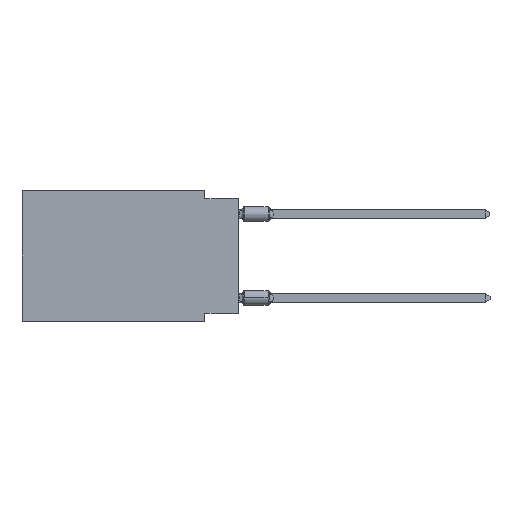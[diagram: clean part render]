
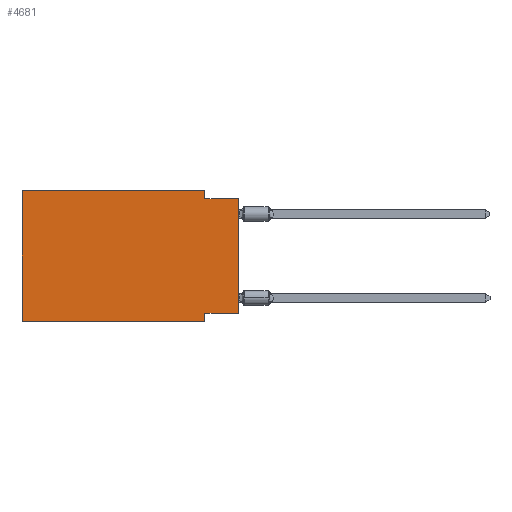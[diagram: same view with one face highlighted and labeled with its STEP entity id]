
A CAD part, left-side view. The second image highlights one B-rep face of the part: STEP entity #4681.
In plain terms, the highlighted planar face has unit normal (-1, 0, 0).
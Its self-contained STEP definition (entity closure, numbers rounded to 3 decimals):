
#393 = VECTOR ( 'NONE', #967, 1000. ) ;
#500 = DIRECTION ( 'NONE',  ( 0., 1., 0. ) ) ;
#753 = CARTESIAN_POINT ( 'NONE',  ( 0., 2.54, 0. ) ) ;
#770 = VECTOR ( 'NONE', #23218, 1000. ) ;
#847 = LINE ( 'NONE', #4519, #770 ) ;
#901 = CARTESIAN_POINT ( 'NONE',  ( 0., 0., -0.635 ) ) ;
#967 = DIRECTION ( 'NONE',  ( 0., -1., 0. ) ) ;
#1133 = VECTOR ( 'NONE', #22159, 1000. ) ;
#1694 = AXIS2_PLACEMENT_3D ( 'NONE', #12767, #22157, #8851 ) ;
#1802 = ORIENTED_EDGE ( 'NONE', *, *, #13417, .T. ) ;
#1824 = VECTOR ( 'NONE', #11027, 1000. ) ;
#2027 = ORIENTED_EDGE ( 'NONE', *, *, #6627, .F. ) ;
#2348 = LINE ( 'NONE', #753, #22731 ) ;
#2801 = LINE ( 'NONE', #17723, #393 ) ;
#3312 = CARTESIAN_POINT ( 'NONE',  ( 0., 16.383, -9.906 ) ) ;
#3412 = CARTESIAN_POINT ( 'NONE',  ( 0., 2.54, -9.906 ) ) ;
#3560 = CARTESIAN_POINT ( 'NONE',  ( 0., 2.54, 0. ) ) ;
#3595 = ORIENTED_EDGE ( 'NONE', *, *, #3862, .F. ) ;
#3862 = EDGE_CURVE ( 'NONE', #17677, #14740, #12739, .T. ) ;
#4302 = EDGE_CURVE ( 'NONE', #20389, #4439, #18160, .T. ) ;
#4439 = VERTEX_POINT ( 'NONE', #901 ) ;
#4519 = CARTESIAN_POINT ( 'NONE',  ( 0., 0., 0. ) ) ;
#4681 = ADVANCED_FACE ( 'NONE', ( #8731 ), #5280, .F. ) ;
#4986 = VERTEX_POINT ( 'NONE', #3312 ) ;
#5280 = PLANE ( 'NONE',  #1694 ) ;
#5672 = CARTESIAN_POINT ( 'NONE',  ( 0., 0., -0.635 ) ) ;
#6627 = EDGE_CURVE ( 'NONE', #17082, #17677, #20934, .T. ) ;
#7326 = CARTESIAN_POINT ( 'NONE',  ( 0., 2.54, -9.906 ) ) ;
#8063 = ORIENTED_EDGE ( 'NONE', *, *, #4302, .F. ) ;
#8145 = ORIENTED_EDGE ( 'NONE', *, *, #13452, .T. ) ;
#8538 = EDGE_LOOP ( 'NONE', ( #1802, #8063, #15615, #14293, #20192, #8145, #3595, #2027 ) ) ;
#8731 = FACE_OUTER_BOUND ( 'NONE', #8538, .T. ) ;
#8851 = DIRECTION ( 'NONE',  ( 0., 0., -1. ) ) ;
#9338 = CARTESIAN_POINT ( 'NONE',  ( 0., 16.383, 0. ) ) ;
#11027 = DIRECTION ( 'NONE',  ( 0., 0., -1. ) ) ;
#11295 = CARTESIAN_POINT ( 'NONE',  ( 0., 16.383, 0. ) ) ;
#11625 = VECTOR ( 'NONE', #500, 1000. ) ;
#11917 = EDGE_CURVE ( 'NONE', #14291, #20389, #2348, .T. ) ;
#12386 = CARTESIAN_POINT ( 'NONE',  ( 0., 16.383, 0. ) ) ;
#12739 = LINE ( 'NONE', #7326, #1824 ) ;
#12767 = CARTESIAN_POINT ( 'NONE',  ( 0., 16.383, 0. ) ) ;
#13256 = LINE ( 'NONE', #9338, #14439 ) ;
#13417 = EDGE_CURVE ( 'NONE', #17082, #4439, #847, .T. ) ;
#13452 = EDGE_CURVE ( 'NONE', #4986, #14740, #2801, .T. ) ;
#13636 = CARTESIAN_POINT ( 'NONE',  ( 0., 0., -9.271 ) ) ;
#13716 = CARTESIAN_POINT ( 'NONE',  ( 0., 0., -9.271 ) ) ;
#14291 = VERTEX_POINT ( 'NONE', #3560 ) ;
#14293 = ORIENTED_EDGE ( 'NONE', *, *, #17766, .F. ) ;
#14439 = VECTOR ( 'NONE', #22408, 1000. ) ;
#14740 = VERTEX_POINT ( 'NONE', #3412 ) ;
#15547 = VECTOR ( 'NONE', #19020, 1000. ) ;
#15615 = ORIENTED_EDGE ( 'NONE', *, *, #11917, .F. ) ;
#15693 = DIRECTION ( 'NONE',  ( 0., 0., -1. ) ) ;
#16190 = CARTESIAN_POINT ( 'NONE',  ( 0., 2.54, -9.271 ) ) ;
#17082 = VERTEX_POINT ( 'NONE', #13636 ) ;
#17677 = VERTEX_POINT ( 'NONE', #16190 ) ;
#17723 = CARTESIAN_POINT ( 'NONE',  ( 0., 16.383, -9.906 ) ) ;
#17747 = EDGE_CURVE ( 'NONE', #4986, #19350, #13256, .T. ) ;
#17766 = EDGE_CURVE ( 'NONE', #19350, #14291, #22279, .T. ) ;
#18160 = LINE ( 'NONE', #5672, #15547 ) ;
#19020 = DIRECTION ( 'NONE',  ( 0., -1., 0. ) ) ;
#19350 = VERTEX_POINT ( 'NONE', #12386 ) ;
#20192 = ORIENTED_EDGE ( 'NONE', *, *, #17747, .F. ) ;
#20389 = VERTEX_POINT ( 'NONE', #21108 ) ;
#20934 = LINE ( 'NONE', #13716, #11625 ) ;
#21108 = CARTESIAN_POINT ( 'NONE',  ( 0., 2.54, -0.635 ) ) ;
#22157 = DIRECTION ( 'NONE',  ( 1., 0., 0. ) ) ;
#22159 = DIRECTION ( 'NONE',  ( 0., -1., 0. ) ) ;
#22279 = LINE ( 'NONE', #11295, #1133 ) ;
#22408 = DIRECTION ( 'NONE',  ( 0., 0., 1. ) ) ;
#22731 = VECTOR ( 'NONE', #15693, 1000. ) ;
#23218 = DIRECTION ( 'NONE',  ( 0., 0., 1. ) ) ;
